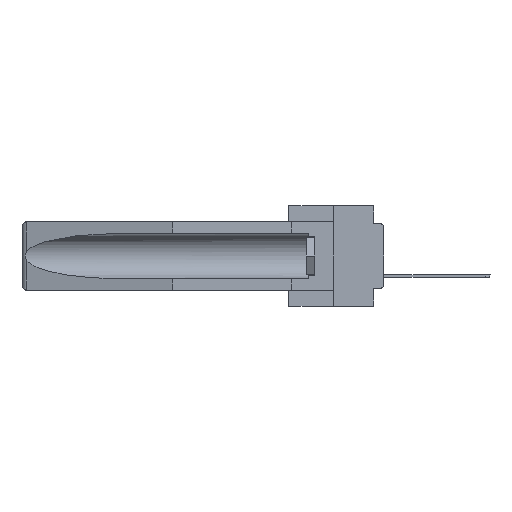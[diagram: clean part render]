
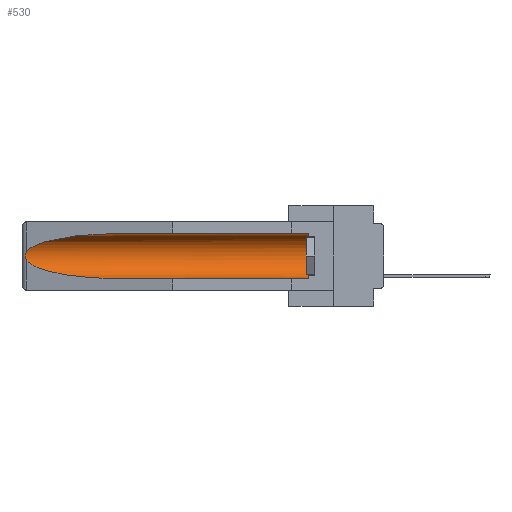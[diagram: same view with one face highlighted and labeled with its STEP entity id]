
A CAD part, left-side view. The second image highlights one B-rep face of the part: STEP entity #530.
In plain terms, the highlighted cylindrical face has radius 2.857 mm (diameter 5.715 mm), a partial arc.
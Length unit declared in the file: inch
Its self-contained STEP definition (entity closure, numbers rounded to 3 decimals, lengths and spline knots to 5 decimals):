
#530 = ADVANCED_FACE ( 'NONE', ( #14734 ), #12944, .F. ) ;
#806 = VERTEX_POINT ( 'NONE', #30088 ) ;
#1819 = VECTOR ( 'NONE', #7541, 39.37008 ) ;
#1991 = CARTESIAN_POINT ( 'NONE',  ( 0.26537, 1.52718, -0.19328 ) ) ;
#2632 = EDGE_CURVE ( 'NONE', #26420, #29048, #26751, .T. ) ;
#3721 = B_SPLINE_CURVE_WITH_KNOTS ( 'NONE', 3,
 ( #17811, #6329, #27663, #11271, #29696, #3761, #11070, #20287, #22630, #17911 ),
 .UNSPECIFIED., .F., .F.,
 ( 4, 2, 2, 2, 4 ),
 ( 0., 0.00029, 0.00058, 0.00087, 0.00117 ),
 .UNSPECIFIED. ) ;
#3761 = CARTESIAN_POINT ( 'NONE',  ( 0.2675, 1.53308, -0.17534 ) ) ;
#3894 = ORIENTED_EDGE ( 'NONE', *, *, #18160, .T. ) ;
#4457 = DIRECTION ( 'NONE',  ( 0., 0., 1. ) ) ;
#4852 = CARTESIAN_POINT ( 'NONE',  ( 0.155, -0.30754, -0.059 ) ) ;
#5147 = ORIENTED_EDGE ( 'NONE', *, *, #15382, .T. ) ;
#5272 = EDGE_CURVE ( 'NONE', #29048, #806, #24596, .T. ) ;
#5738 = ORIENTED_EDGE ( 'NONE', *, *, #10759, .F. ) ;
#6329 = CARTESIAN_POINT ( 'NONE',  ( 0.26597, 1.52961, -0.15275 ) ) ;
#7541 = DIRECTION ( 'NONE',  ( 0., 1., 0. ) ) ;
#7647 = VECTOR ( 'NONE', #12773, 39.37008 ) ;
#9703 = DIRECTION ( 'NONE',  ( 0., 0., 1. ) ) ;
#10369 = CARTESIAN_POINT ( 'NONE',  ( 0.155, 1.07973, -0.284 ) ) ;
#10759 = EDGE_CURVE ( 'NONE', #28428, #28877, #30363, .T. ) ;
#10999 = AXIS2_PLACEMENT_3D ( 'NONE', #16050, #28055, #9703 ) ;
#11070 = CARTESIAN_POINT ( 'NONE',  ( 0.2673, 1.53269, -0.17917 ) ) ;
#11271 = CARTESIAN_POINT ( 'NONE',  ( 0.2673, 1.5327, -0.16383 ) ) ;
#11729 = VERTEX_POINT ( 'NONE', #13639 ) ;
#11910 = CARTESIAN_POINT ( 'NONE',  ( 0.21114, 1.30732, -0.284 ) ) ;
#12773 = DIRECTION ( 'NONE',  ( 0., 1., 0. ) ) ;
#12944 = CYLINDRICAL_SURFACE ( 'NONE', #10999, 0.1125 ) ;
#12999 = AXIS2_PLACEMENT_3D ( 'NONE', #16558, #25701, #4457 ) ;
#13639 = CARTESIAN_POINT ( 'NONE',  ( 0.26537, 1.52718, -0.19328 ) ) ;
#14734 = FACE_OUTER_BOUND ( 'NONE', #22914, .T. ) ;
#14965 = CARTESIAN_POINT ( 'NONE',  ( 0.26537, 1.52718, -0.14972 ) ) ;
#15283 = ORIENTED_EDGE ( 'NONE', *, *, #17897, .T. ) ;
#15382 = EDGE_CURVE ( 'NONE', #11729, #28877, #28687, .T. ) ;
#16050 = CARTESIAN_POINT ( 'NONE',  ( 0.155, -0.30754, -0.1715 ) ) ;
#16558 = CARTESIAN_POINT ( 'NONE',  ( 0.155, 0.126, -0.1715 ) ) ;
#17357 = CARTESIAN_POINT ( 'NONE',  ( 0.21114, 1.30732, -0.059 ) ) ;
#17811 = CARTESIAN_POINT ( 'NONE',  ( 0.26537, 1.52718, -0.14972 ) ) ;
#17840 = CARTESIAN_POINT ( 'NONE',  ( 0.155, 1.07973, -0.059 ) ) ;
#17897 = EDGE_CURVE ( 'NONE', #28428, #26420, #29297, .T. ) ;
#17911 = CARTESIAN_POINT ( 'NONE',  ( 0.26537, 1.52718, -0.19328 ) ) ;
#18160 = EDGE_CURVE ( 'NONE', #806, #11729, #3721, .T. ) ;
#18374 = CARTESIAN_POINT ( 'NONE',  ( 0.155, 0.126, -0.284 ) ) ;
#20287 = CARTESIAN_POINT ( 'NONE',  ( 0.26655, 1.53094, -0.18657 ) ) ;
#20737 = CARTESIAN_POINT ( 'NONE',  ( 0.25451, 1.48313, -0.24835 ) ) ;
#21443 = CARTESIAN_POINT ( 'NONE',  ( 0.155, 1.07973, -0.059 ) ) ;
#22630 = CARTESIAN_POINT ( 'NONE',  ( 0.26597, 1.5296, -0.19026 ) ) ;
#22914 = EDGE_LOOP ( 'NONE', ( #28086, #3894, #5147, #5738, #15283, #26883 ) ) ;
#23783 = CARTESIAN_POINT ( 'NONE',  ( 0.155, 1.07973, -0.284 ) ) ;
#24567 = CARTESIAN_POINT ( 'NONE',  ( 0.155, -0.30754, -0.284 ) ) ;
#24596 =( BOUNDED_CURVE ( )  B_SPLINE_CURVE ( 3, ( #21443, #17357, #29017, #14965 ),
 .UNSPECIFIED., .F., .F. ) 
 B_SPLINE_CURVE_WITH_KNOTS ( ( 4, 4 ),
 ( 4.71239, 6.08839 ),
 .UNSPECIFIED. ) 
 CURVE ( )  GEOMETRIC_REPRESENTATION_ITEM ( )  RATIONAL_B_SPLINE_CURVE ( ( 1., 0.848, 0.848, 1. ) ) 
 REPRESENTATION_ITEM ( '' )  );
#25701 = DIRECTION ( 'NONE',  ( 0., -1., 0. ) ) ;
#26420 = VERTEX_POINT ( 'NONE', #26993 ) ;
#26751 = LINE ( 'NONE', #4852, #1819 ) ;
#26883 = ORIENTED_EDGE ( 'NONE', *, *, #2632, .T. ) ;
#26993 = CARTESIAN_POINT ( 'NONE',  ( 0.155, 0.126, -0.059 ) ) ;
#27663 = CARTESIAN_POINT ( 'NONE',  ( 0.26654, 1.53092, -0.15636 ) ) ;
#28055 = DIRECTION ( 'NONE',  ( 0., 1., 0. ) ) ;
#28086 = ORIENTED_EDGE ( 'NONE', *, *, #5272, .T. ) ;
#28428 = VERTEX_POINT ( 'NONE', #18374 ) ;
#28687 =( BOUNDED_CURVE ( )  B_SPLINE_CURVE ( 3, ( #1991, #20737, #11910, #23783 ),
 .UNSPECIFIED., .F., .F. ) 
 B_SPLINE_CURVE_WITH_KNOTS ( ( 4, 4 ),
 ( 0.1948, 1.5708 ),
 .UNSPECIFIED. ) 
 CURVE ( )  GEOMETRIC_REPRESENTATION_ITEM ( )  RATIONAL_B_SPLINE_CURVE ( ( 1., 0.848, 0.848, 1. ) ) 
 REPRESENTATION_ITEM ( '' )  );
#28877 = VERTEX_POINT ( 'NONE', #10369 ) ;
#29017 = CARTESIAN_POINT ( 'NONE',  ( 0.25451, 1.48313, -0.09465 ) ) ;
#29048 = VERTEX_POINT ( 'NONE', #17840 ) ;
#29297 = CIRCLE ( 'NONE', #12999, 0.1125 ) ;
#29696 = CARTESIAN_POINT ( 'NONE',  ( 0.2675, 1.53308, -0.16763 ) ) ;
#30088 = CARTESIAN_POINT ( 'NONE',  ( 0.26537, 1.52718, -0.14972 ) ) ;
#30363 = LINE ( 'NONE', #24567, #7647 ) ;
